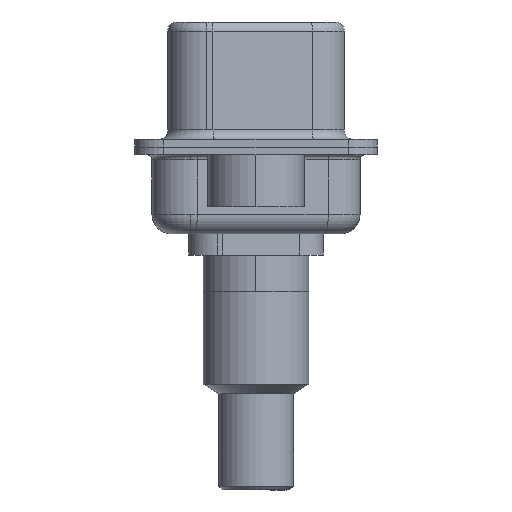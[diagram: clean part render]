
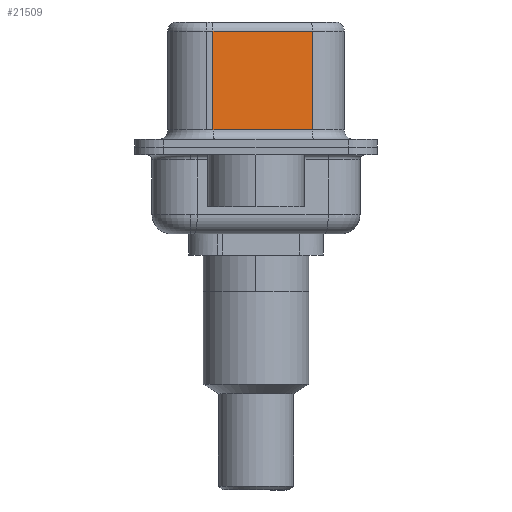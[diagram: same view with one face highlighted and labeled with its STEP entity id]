
A CAD part, left-side view. The second image highlights one B-rep face of the part: STEP entity #21509.
In plain terms, the highlighted planar face has unit normal (-0.985, -0.174, 0).
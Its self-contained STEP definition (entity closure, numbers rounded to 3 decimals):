
#400 = CARTESIAN_POINT ( 'NONE',  ( 4.565, -2.927, 6.02 ) ) ;
#703 = ORIENTED_EDGE ( 'NONE', *, *, #1751, .T. ) ;
#1725 = VECTOR ( 'NONE', #21524, 1000. ) ;
#1751 = EDGE_CURVE ( 'NONE', #13408, #7220, #22123, .T. ) ;
#2085 = DIRECTION ( 'NONE',  ( 0., 0., -1. ) ) ;
#2909 = VECTOR ( 'NONE', #11277, 1000. ) ;
#2928 = PLANE ( 'NONE',  #15658 ) ;
#3546 = VERTEX_POINT ( 'NONE', #5461 ) ;
#4236 = VECTOR ( 'NONE', #2085, 1000. ) ;
#4560 = ORIENTED_EDGE ( 'NONE', *, *, #6893, .F. ) ;
#4727 = DIRECTION ( 'NONE',  ( -0.174, 0.985, 0. ) ) ;
#5461 = CARTESIAN_POINT ( 'NONE',  ( 4.565, -2.927, 6.02 ) ) ;
#5962 = LINE ( 'NONE', #21626, #1725 ) ;
#6579 = EDGE_CURVE ( 'NONE', #7220, #6697, #10136, .T. ) ;
#6697 = VERTEX_POINT ( 'NONE', #16329 ) ;
#6893 = EDGE_CURVE ( 'NONE', #3546, #6697, #5962, .T. ) ;
#7220 = VERTEX_POINT ( 'NONE', #9010 ) ;
#9010 = CARTESIAN_POINT ( 'NONE',  ( 3.655, 2.233, 0.9 ) ) ;
#10136 = LINE ( 'NONE', #10917, #23079 ) ;
#10917 = CARTESIAN_POINT ( 'NONE',  ( 4.565, -2.927, 0.9 ) ) ;
#10999 = DIRECTION ( 'NONE',  ( 0.174, -0.985, 0. ) ) ;
#11277 = DIRECTION ( 'NONE',  ( -0.174, 0.985, 0. ) ) ;
#11335 = CARTESIAN_POINT ( 'NONE',  ( 3.655, 2.233, 6.52 ) ) ;
#11799 = EDGE_CURVE ( 'NONE', #3546, #13408, #13775, .T. ) ;
#13408 = VERTEX_POINT ( 'NONE', #20066 ) ;
#13775 = LINE ( 'NONE', #400, #2909 ) ;
#13792 = CARTESIAN_POINT ( 'NONE',  ( 4.565, -2.927, 6.52 ) ) ;
#15118 = ORIENTED_EDGE ( 'NONE', *, *, #11799, .T. ) ;
#15621 = DIRECTION ( 'NONE',  ( 0.985, 0.174, 0. ) ) ;
#15658 = AXIS2_PLACEMENT_3D ( 'NONE', #13792, #15621, #4727 ) ;
#16329 = CARTESIAN_POINT ( 'NONE',  ( 4.565, -2.927, 0.9 ) ) ;
#17016 = ORIENTED_EDGE ( 'NONE', *, *, #6579, .T. ) ;
#18056 = FACE_OUTER_BOUND ( 'NONE', #22934, .T. ) ;
#20066 = CARTESIAN_POINT ( 'NONE',  ( 3.655, 2.233, 6.02 ) ) ;
#21509 = ADVANCED_FACE ( 'NONE', ( #18056 ), #2928, .F. ) ;
#21524 = DIRECTION ( 'NONE',  ( 0., 0., -1. ) ) ;
#21626 = CARTESIAN_POINT ( 'NONE',  ( 4.565, -2.927, 6.52 ) ) ;
#22123 = LINE ( 'NONE', #11335, #4236 ) ;
#22934 = EDGE_LOOP ( 'NONE', ( #4560, #15118, #703, #17016 ) ) ;
#23079 = VECTOR ( 'NONE', #10999, 1000. ) ;
